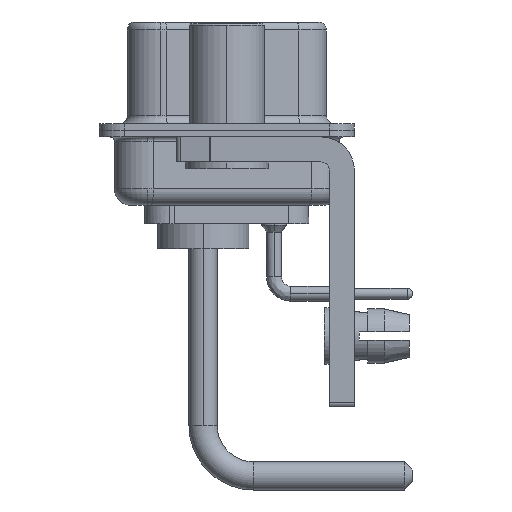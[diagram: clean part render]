
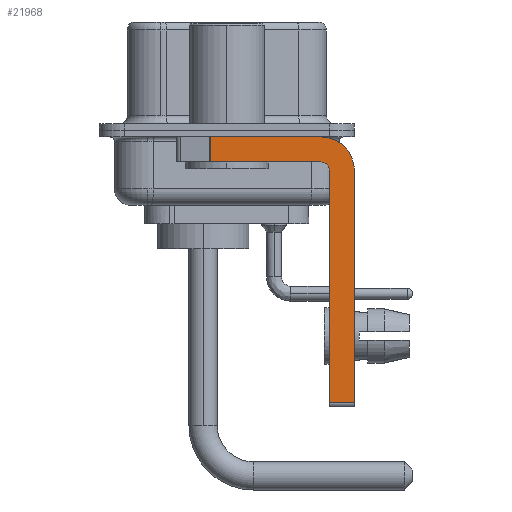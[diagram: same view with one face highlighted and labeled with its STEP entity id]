
A CAD part, left-side view. The second image highlights one B-rep face of the part: STEP entity #21968.
In plain terms, the highlighted planar face has unit normal (-1, 0, 0).
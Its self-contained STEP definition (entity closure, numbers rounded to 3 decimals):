
#158 = VECTOR ( 'NONE', #14747, 1000. ) ;
#659 = AXIS2_PLACEMENT_3D ( 'NONE', #5277, #5412, #22686 ) ;
#1578 = EDGE_LOOP ( 'NONE', ( #12346, #12586, #23613, #22602, #7029, #12018, #5332, #11067 ) ) ;
#1586 = DIRECTION ( 'NONE',  ( 0., 0., 1. ) ) ;
#2337 = VERTEX_POINT ( 'NONE', #8183 ) ;
#3665 = EDGE_CURVE ( 'NONE', #5125, #11879, #16608, .T. ) ;
#4369 = CARTESIAN_POINT ( 'NONE',  ( -2.9, -7.65, -2.4 ) ) ;
#4692 = EDGE_CURVE ( 'NONE', #26237, #24002, #25432, .T. ) ;
#5125 = VERTEX_POINT ( 'NONE', #22991 ) ;
#5277 = CARTESIAN_POINT ( 'NONE',  ( -2.9, -5.65, -2.4 ) ) ;
#5317 = DIRECTION ( 'NONE',  ( 0., 0., 1. ) ) ;
#5332 = ORIENTED_EDGE ( 'NONE', *, *, #16338, .F. ) ;
#5412 = DIRECTION ( 'NONE',  ( 1., 0., 0. ) ) ;
#5770 = VECTOR ( 'NONE', #14391, 1000. ) ;
#6582 = DIRECTION ( 'NONE',  ( 0., 0., -1. ) ) ;
#7029 = ORIENTED_EDGE ( 'NONE', *, *, #3665, .F. ) ;
#7046 = CARTESIAN_POINT ( 'NONE',  ( -2.9, -6.15, -2.4 ) ) ;
#7397 = FACE_OUTER_BOUND ( 'NONE', #1578, .T. ) ;
#8099 = LINE ( 'NONE', #19116, #158 ) ;
#8183 = CARTESIAN_POINT ( 'NONE',  ( -2.9, -5.65, -1.9 ) ) ;
#8466 = CIRCLE ( 'NONE', #14816, 2. ) ;
#9148 = VECTOR ( 'NONE', #1586, 1000. ) ;
#10529 = EDGE_CURVE ( 'NONE', #26237, #22664, #27943, .T. ) ;
#11015 = DIRECTION ( 'NONE',  ( 0., 0., -1. ) ) ;
#11067 = ORIENTED_EDGE ( 'NONE', *, *, #25853, .F. ) ;
#11879 = VERTEX_POINT ( 'NONE', #7046 ) ;
#12018 = ORIENTED_EDGE ( 'NONE', *, *, #15371, .T. ) ;
#12094 = VERTEX_POINT ( 'NONE', #25831 ) ;
#12346 = ORIENTED_EDGE ( 'NONE', *, *, #4692, .F. ) ;
#12427 = CIRCLE ( 'NONE', #25079, 0.5 ) ;
#12586 = ORIENTED_EDGE ( 'NONE', *, *, #10529, .T. ) ;
#14058 = PLANE ( 'NONE',  #659 ) ;
#14391 = DIRECTION ( 'NONE',  ( 0., -1., 0. ) ) ;
#14430 = EDGE_CURVE ( 'NONE', #2337, #22664, #8099, .T. ) ;
#14747 = DIRECTION ( 'NONE',  ( 0., 1., 0. ) ) ;
#14816 = AXIS2_PLACEMENT_3D ( 'NONE', #15794, #20172, #6582 ) ;
#15190 = EDGE_CURVE ( 'NONE', #11879, #2337, #12427, .T. ) ;
#15371 = EDGE_CURVE ( 'NONE', #5125, #20651, #25418, .T. ) ;
#15794 = CARTESIAN_POINT ( 'NONE',  ( -2.9, -5.65, -2.4 ) ) ;
#16338 = EDGE_CURVE ( 'NONE', #12094, #20651, #26052, .T. ) ;
#16494 = CARTESIAN_POINT ( 'NONE',  ( -2.9, -5.65, -2.4 ) ) ;
#16608 = LINE ( 'NONE', #21131, #9148 ) ;
#16637 = DIRECTION ( 'NONE',  ( -1., 0., 0. ) ) ;
#16904 = DIRECTION ( 'NONE',  ( 0., -1., 0. ) ) ;
#17156 = CARTESIAN_POINT ( 'NONE',  ( -2.9, 0.978, -1.9 ) ) ;
#18736 = CARTESIAN_POINT ( 'NONE',  ( -2.9, -7.65, -16.35 ) ) ;
#19116 = CARTESIAN_POINT ( 'NONE',  ( -2.9, -5.65, -1.9 ) ) ;
#19499 = VECTOR ( 'NONE', #21550, 1000. ) ;
#20172 = DIRECTION ( 'NONE',  ( 1., 0., 0. ) ) ;
#20651 = VERTEX_POINT ( 'NONE', #18736 ) ;
#21131 = CARTESIAN_POINT ( 'NONE',  ( -2.9, -6.15, -16.6 ) ) ;
#21550 = DIRECTION ( 'NONE',  ( 0., 0., -1. ) ) ;
#21968 = ADVANCED_FACE ( 'NONE', ( #7397 ), #14058, .F. ) ;
#22602 = ORIENTED_EDGE ( 'NONE', *, *, #15190, .F. ) ;
#22664 = VERTEX_POINT ( 'NONE', #26011 ) ;
#22686 = DIRECTION ( 'NONE',  ( 0., 0., -1. ) ) ;
#22991 = CARTESIAN_POINT ( 'NONE',  ( -2.9, -6.15, -16.35 ) ) ;
#23613 = ORIENTED_EDGE ( 'NONE', *, *, #14430, .F. ) ;
#24002 = VERTEX_POINT ( 'NONE', #25914 ) ;
#24185 = VECTOR ( 'NONE', #16904, 1000. ) ;
#25079 = AXIS2_PLACEMENT_3D ( 'NONE', #16494, #16637, #5317 ) ;
#25418 = LINE ( 'NONE', #27551, #24185 ) ;
#25432 = LINE ( 'NONE', #27284, #5770 ) ;
#25831 = CARTESIAN_POINT ( 'NONE',  ( -2.9, -7.65, -2.4 ) ) ;
#25853 = EDGE_CURVE ( 'NONE', #24002, #12094, #8466, .T. ) ;
#25914 = CARTESIAN_POINT ( 'NONE',  ( -2.9, -5.65, -0.4 ) ) ;
#26011 = CARTESIAN_POINT ( 'NONE',  ( -2.9, 0.978, -1.9 ) ) ;
#26052 = LINE ( 'NONE', #4369, #26940 ) ;
#26237 = VERTEX_POINT ( 'NONE', #26356 ) ;
#26356 = CARTESIAN_POINT ( 'NONE',  ( -2.9, 0.978, -0.4 ) ) ;
#26940 = VECTOR ( 'NONE', #11015, 1000. ) ;
#27284 = CARTESIAN_POINT ( 'NONE',  ( -2.9, 3., -0.4 ) ) ;
#27551 = CARTESIAN_POINT ( 'NONE',  ( -2.9, -5.65, -16.35 ) ) ;
#27943 = LINE ( 'NONE', #17156, #19499 ) ;
